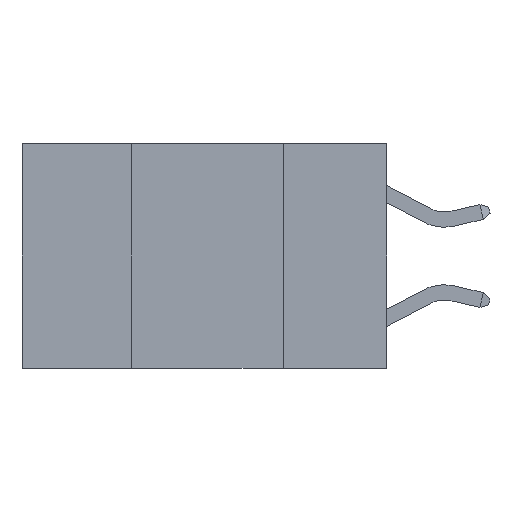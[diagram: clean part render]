
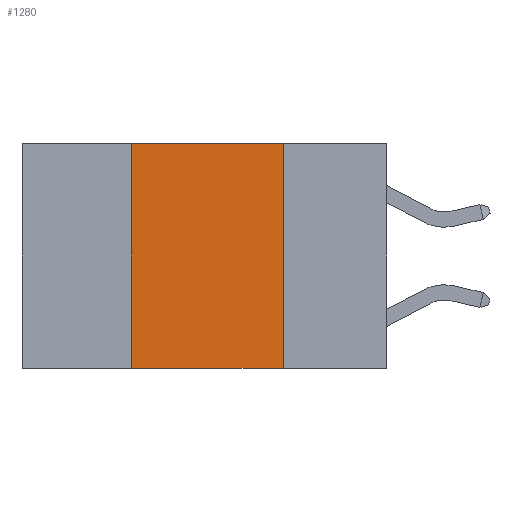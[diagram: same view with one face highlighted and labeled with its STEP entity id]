
A CAD part, left-side view. The second image highlights one B-rep face of the part: STEP entity #1280.
In plain terms, the highlighted planar face has unit normal (-1, 0, 0).
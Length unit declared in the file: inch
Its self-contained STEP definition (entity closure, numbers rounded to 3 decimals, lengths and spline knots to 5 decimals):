
#3 = CARTESIAN_POINT ( 'NONE',  ( 0., 0.17, -0.37 ) ) ;
#35 = VECTOR ( 'NONE', #8438, 39.37008 ) ;
#319 = LINE ( 'NONE', #7546, #35 ) ;
#451 = EDGE_CURVE ( 'NONE', #3494, #4445, #3119, .T. ) ;
#1047 = EDGE_CURVE ( 'NONE', #8697, #6497, #2647, .T. ) ;
#1050 = EDGE_CURVE ( 'NONE', #4445, #6497, #319, .T. ) ;
#1091 = EDGE_CURVE ( 'NONE', #8697, #3494, #2396, .T. ) ;
#1280 = ADVANCED_FACE ( 'NONE', ( #2112 ), #5377, .F. ) ;
#2112 = FACE_OUTER_BOUND ( 'NONE', #5345, .T. ) ;
#2396 = LINE ( 'NONE', #4642, #5871 ) ;
#2647 = LINE ( 'NONE', #3392, #2862 ) ;
#2862 = VECTOR ( 'NONE', #3763, 39.37008 ) ;
#3119 = LINE ( 'NONE', #4619, #4601 ) ;
#3392 = CARTESIAN_POINT ( 'NONE',  ( 0., 0.6, -0.37 ) ) ;
#3494 = VERTEX_POINT ( 'NONE', #9052 ) ;
#3763 = DIRECTION ( 'NONE',  ( 0., -1., 0. ) ) ;
#4361 = ORIENTED_EDGE ( 'NONE', *, *, #1050, .F. ) ;
#4445 = VERTEX_POINT ( 'NONE', #6435 ) ;
#4601 = VECTOR ( 'NONE', #9909, 39.37008 ) ;
#4619 = CARTESIAN_POINT ( 'NONE',  ( 0., 0.6, 0. ) ) ;
#4642 = CARTESIAN_POINT ( 'NONE',  ( 0., 0.42, 0. ) ) ;
#4664 = ORIENTED_EDGE ( 'NONE', *, *, #1047, .T. ) ;
#5297 = CARTESIAN_POINT ( 'NONE',  ( 0., 0.42, -0.37 ) ) ;
#5307 = AXIS2_PLACEMENT_3D ( 'NONE', #5963, #5965, #7753 ) ;
#5345 = EDGE_LOOP ( 'NONE', ( #4361, #8470, #7039, #4664 ) ) ;
#5377 = PLANE ( 'NONE',  #5307 ) ;
#5871 = VECTOR ( 'NONE', #7662, 39.37008 ) ;
#5963 = CARTESIAN_POINT ( 'NONE',  ( 0., 0.6, 0. ) ) ;
#5965 = DIRECTION ( 'NONE',  ( 1., 0., 0. ) ) ;
#6435 = CARTESIAN_POINT ( 'NONE',  ( 0., 0.17, 0. ) ) ;
#6497 = VERTEX_POINT ( 'NONE', #3 ) ;
#7039 = ORIENTED_EDGE ( 'NONE', *, *, #1091, .F. ) ;
#7546 = CARTESIAN_POINT ( 'NONE',  ( 0., 0.17, 0. ) ) ;
#7662 = DIRECTION ( 'NONE',  ( 0., 0., 1. ) ) ;
#7753 = DIRECTION ( 'NONE',  ( 0., 0., -1. ) ) ;
#8438 = DIRECTION ( 'NONE',  ( 0., 0., -1. ) ) ;
#8470 = ORIENTED_EDGE ( 'NONE', *, *, #451, .F. ) ;
#8697 = VERTEX_POINT ( 'NONE', #5297 ) ;
#9052 = CARTESIAN_POINT ( 'NONE',  ( 0., 0.42, 0. ) ) ;
#9909 = DIRECTION ( 'NONE',  ( 0., -1., 0. ) ) ;
